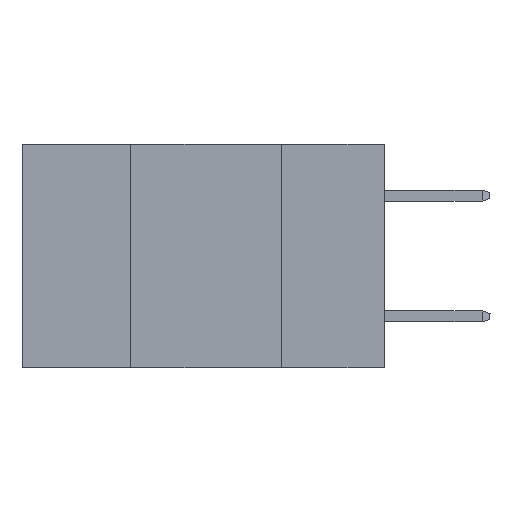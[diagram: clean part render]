
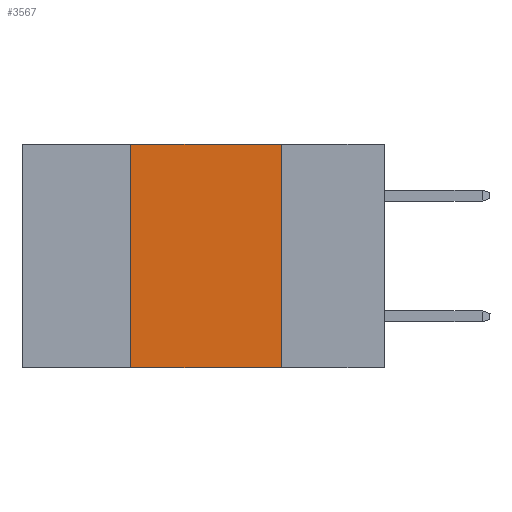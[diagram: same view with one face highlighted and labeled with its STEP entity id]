
A CAD part, left-side view. The second image highlights one B-rep face of the part: STEP entity #3567.
In plain terms, the highlighted planar face has unit normal (-1, 0, 0).
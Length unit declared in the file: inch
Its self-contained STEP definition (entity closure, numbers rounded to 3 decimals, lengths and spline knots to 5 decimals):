
#803 = EDGE_LOOP ( 'NONE', ( #16260, #2990, #2457, #10883 ) ) ;
#993 = CARTESIAN_POINT ( 'NONE',  ( 0., 0.42, 0. ) ) ;
#1921 = DIRECTION ( 'NONE',  ( 0., -1., 0. ) ) ;
#2457 = ORIENTED_EDGE ( 'NONE', *, *, #7237, .F. ) ;
#2571 = VECTOR ( 'NONE', #1921, 39.37008 ) ;
#2687 = DIRECTION ( 'NONE',  ( 0., 0., 1. ) ) ;
#2990 = ORIENTED_EDGE ( 'NONE', *, *, #10093, .F. ) ;
#3567 = ADVANCED_FACE ( 'NONE', ( #7655 ), #13924, .F. ) ;
#4730 = VECTOR ( 'NONE', #2687, 39.37008 ) ;
#4918 = CARTESIAN_POINT ( 'NONE',  ( 0., 0.17, 0. ) ) ;
#5446 = DIRECTION ( 'NONE',  ( 0., 0., -1. ) ) ;
#6059 = EDGE_CURVE ( 'NONE', #9341, #9013, #13176, .T. ) ;
#7237 = EDGE_CURVE ( 'NONE', #9341, #15018, #8126, .T. ) ;
#7241 = CARTESIAN_POINT ( 'NONE',  ( 0., 0.6, 0. ) ) ;
#7655 = FACE_OUTER_BOUND ( 'NONE', #803, .T. ) ;
#8126 = LINE ( 'NONE', #14053, #4730 ) ;
#8652 = DIRECTION ( 'NONE',  ( 0., 0., -1. ) ) ;
#8815 = CARTESIAN_POINT ( 'NONE',  ( 0., 0.6, 0. ) ) ;
#9013 = VERTEX_POINT ( 'NONE', #15690 ) ;
#9341 = VERTEX_POINT ( 'NONE', #14589 ) ;
#9743 = DIRECTION ( 'NONE',  ( 0., -1., 0. ) ) ;
#9968 = EDGE_CURVE ( 'NONE', #15021, #9013, #10284, .T. ) ;
#10093 = EDGE_CURVE ( 'NONE', #15018, #15021, #11489, .T. ) ;
#10284 = LINE ( 'NONE', #15576, #11693 ) ;
#10883 = ORIENTED_EDGE ( 'NONE', *, *, #6059, .T. ) ;
#10901 = VECTOR ( 'NONE', #9743, 39.37008 ) ;
#11123 = AXIS2_PLACEMENT_3D ( 'NONE', #8815, #11443, #8652 ) ;
#11443 = DIRECTION ( 'NONE',  ( 1., 0., 0. ) ) ;
#11489 = LINE ( 'NONE', #7241, #10901 ) ;
#11693 = VECTOR ( 'NONE', #5446, 39.37008 ) ;
#13176 = LINE ( 'NONE', #15814, #2571 ) ;
#13924 = PLANE ( 'NONE',  #11123 ) ;
#14053 = CARTESIAN_POINT ( 'NONE',  ( 0., 0.42, 0. ) ) ;
#14589 = CARTESIAN_POINT ( 'NONE',  ( 0., 0.42, -0.37 ) ) ;
#15018 = VERTEX_POINT ( 'NONE', #993 ) ;
#15021 = VERTEX_POINT ( 'NONE', #4918 ) ;
#15576 = CARTESIAN_POINT ( 'NONE',  ( 0., 0.17, 0. ) ) ;
#15690 = CARTESIAN_POINT ( 'NONE',  ( 0., 0.17, -0.37 ) ) ;
#15814 = CARTESIAN_POINT ( 'NONE',  ( 0., 0.6, -0.37 ) ) ;
#16260 = ORIENTED_EDGE ( 'NONE', *, *, #9968, .F. ) ;
